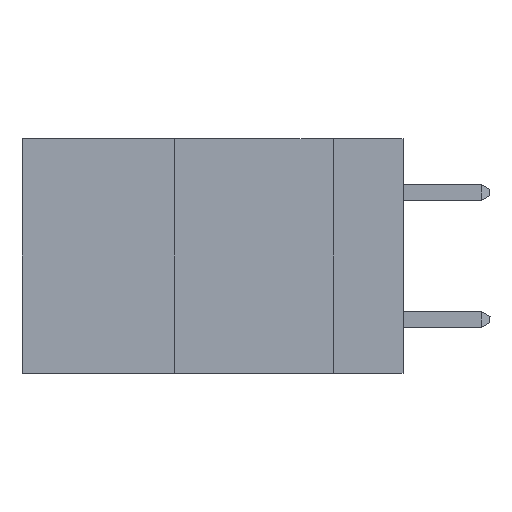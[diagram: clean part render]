
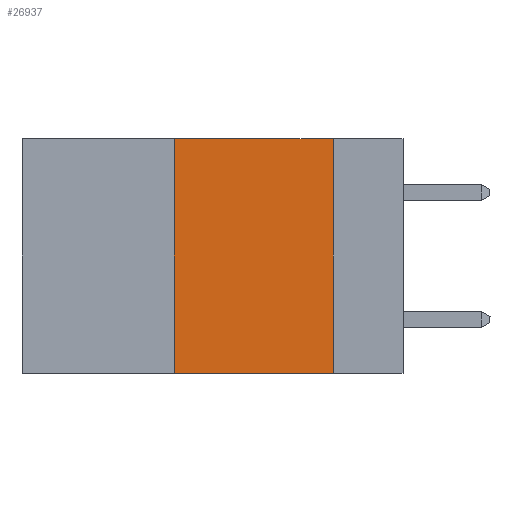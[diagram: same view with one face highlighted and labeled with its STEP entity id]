
A CAD part, left-side view. The second image highlights one B-rep face of the part: STEP entity #26937.
In plain terms, the highlighted planar face has unit normal (-1, 0, 0).
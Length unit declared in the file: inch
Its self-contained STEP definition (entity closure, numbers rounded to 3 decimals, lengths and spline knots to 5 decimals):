
#179 = DIRECTION ( 'NONE',  ( 0., 0., -1. ) ) ;
#1069 = CARTESIAN_POINT ( 'NONE',  ( 0., 0.6, 0. ) ) ;
#1210 = CARTESIAN_POINT ( 'NONE',  ( 0., 0.11, 0. ) ) ;
#1482 = ORIENTED_EDGE ( 'NONE', *, *, #5834, .F. ) ;
#1833 = ORIENTED_EDGE ( 'NONE', *, *, #14215, .F. ) ;
#2448 = VECTOR ( 'NONE', #12173, 39.37008 ) ;
#2977 = AXIS2_PLACEMENT_3D ( 'NONE', #8746, #23659, #179 ) ;
#3755 = VECTOR ( 'NONE', #17832, 39.37008 ) ;
#3905 = CARTESIAN_POINT ( 'NONE',  ( 0., 0.11, 0. ) ) ;
#5834 = EDGE_CURVE ( 'NONE', #15478, #23359, #21764, .T. ) ;
#7322 = LINE ( 'NONE', #21082, #16276 ) ;
#8673 = VERTEX_POINT ( 'NONE', #20942 ) ;
#8746 = CARTESIAN_POINT ( 'NONE',  ( 0., 0.6, 0. ) ) ;
#9448 = EDGE_CURVE ( 'NONE', #18237, #23359, #11024, .T. ) ;
#9454 = EDGE_LOOP ( 'NONE', ( #1482, #1833, #26038, #18550 ) ) ;
#9716 = CARTESIAN_POINT ( 'NONE',  ( 0., 0.11, -0.37 ) ) ;
#11024 = LINE ( 'NONE', #18263, #2448 ) ;
#12173 = DIRECTION ( 'NONE',  ( 0., -1., 0. ) ) ;
#12697 = DIRECTION ( 'NONE',  ( 0., 0., 1. ) ) ;
#14215 = EDGE_CURVE ( 'NONE', #8673, #15478, #14978, .T. ) ;
#14887 = EDGE_CURVE ( 'NONE', #18237, #8673, #7322, .T. ) ;
#14978 = LINE ( 'NONE', #1069, #3755 ) ;
#15478 = VERTEX_POINT ( 'NONE', #1210 ) ;
#16276 = VECTOR ( 'NONE', #12697, 39.37008 ) ;
#17832 = DIRECTION ( 'NONE',  ( 0., -1., 0. ) ) ;
#18237 = VERTEX_POINT ( 'NONE', #26148 ) ;
#18263 = CARTESIAN_POINT ( 'NONE',  ( 0., 0.6, -0.37 ) ) ;
#18287 = DIRECTION ( 'NONE',  ( 0., 0., -1. ) ) ;
#18550 = ORIENTED_EDGE ( 'NONE', *, *, #9448, .T. ) ;
#20942 = CARTESIAN_POINT ( 'NONE',  ( 0., 0.36, 0. ) ) ;
#21082 = CARTESIAN_POINT ( 'NONE',  ( 0., 0.36, 0. ) ) ;
#21431 = VECTOR ( 'NONE', #18287, 39.37008 ) ;
#21488 = PLANE ( 'NONE',  #2977 ) ;
#21764 = LINE ( 'NONE', #3905, #21431 ) ;
#23359 = VERTEX_POINT ( 'NONE', #9716 ) ;
#23659 = DIRECTION ( 'NONE',  ( 1., 0., 0. ) ) ;
#26038 = ORIENTED_EDGE ( 'NONE', *, *, #14887, .F. ) ;
#26148 = CARTESIAN_POINT ( 'NONE',  ( 0., 0.36, -0.37 ) ) ;
#26882 = FACE_OUTER_BOUND ( 'NONE', #9454, .T. ) ;
#26937 = ADVANCED_FACE ( 'NONE', ( #26882 ), #21488, .F. ) ;
